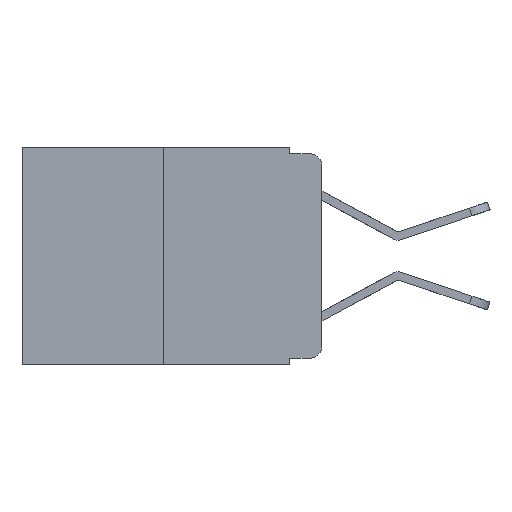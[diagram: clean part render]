
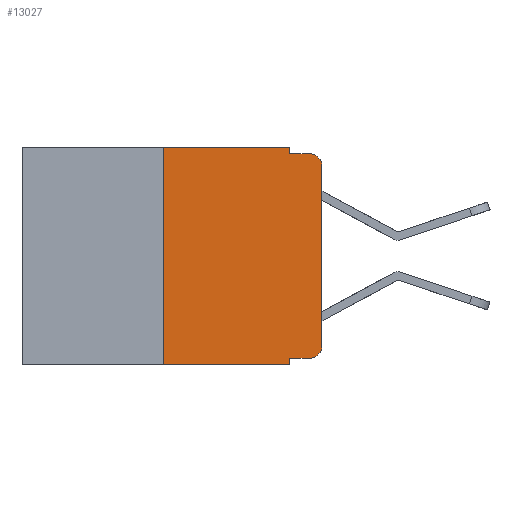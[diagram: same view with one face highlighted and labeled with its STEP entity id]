
A CAD part, left-side view. The second image highlights one B-rep face of the part: STEP entity #13027.
In plain terms, the highlighted planar face has unit normal (-1, 0, 0).
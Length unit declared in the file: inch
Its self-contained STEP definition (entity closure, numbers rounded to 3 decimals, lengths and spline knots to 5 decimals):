
#155 = DIRECTION ( 'NONE',  ( 0., 0., -1. ) ) ;
#633 = EDGE_CURVE ( 'NONE', #12892, #7925, #18901, .T. ) ;
#988 = CARTESIAN_POINT ( 'NONE',  ( 0., 0.473, 0. ) ) ;
#1203 = CARTESIAN_POINT ( 'NONE',  ( 0., 0., -0.313 ) ) ;
#1258 = LINE ( 'NONE', #5531, #10584 ) ;
#1851 = EDGE_CURVE ( 'NONE', #12892, #17118, #18380, .T. ) ;
#2060 = DIRECTION ( 'NONE',  ( 0., -1., 0. ) ) ;
#2754 = CARTESIAN_POINT ( 'NONE',  ( 0., 0.051, 0. ) ) ;
#2759 = ORIENTED_EDGE ( 'NONE', *, *, #19299, .F. ) ;
#2772 = CARTESIAN_POINT ( 'NONE',  ( 0., 0.051, 0. ) ) ;
#2945 = EDGE_CURVE ( 'NONE', #16185, #15703, #11180, .T. ) ;
#3005 = CARTESIAN_POINT ( 'NONE',  ( 0., 0.02, -0.313 ) ) ;
#3011 = VERTEX_POINT ( 'NONE', #1203 ) ;
#3525 = VECTOR ( 'NONE', #8619, 39.37008 ) ;
#3575 = DIRECTION ( 'NONE',  ( -1., 0., 0. ) ) ;
#3885 = CARTESIAN_POINT ( 'NONE',  ( 0., 0.25, 0. ) ) ;
#3967 = ORIENTED_EDGE ( 'NONE', *, *, #5027, .F. ) ;
#3997 = EDGE_CURVE ( 'NONE', #11371, #7748, #6246, .T. ) ;
#4402 = CARTESIAN_POINT ( 'NONE',  ( 0., 0., 0. ) ) ;
#4403 = CARTESIAN_POINT ( 'NONE',  ( 0., 0.051, -0.333 ) ) ;
#4452 = ORIENTED_EDGE ( 'NONE', *, *, #3997, .F. ) ;
#4563 = DIRECTION ( 'NONE',  ( 0., 0., -1. ) ) ;
#4680 = PLANE ( 'NONE',  #9326 ) ;
#5027 = EDGE_CURVE ( 'NONE', #7748, #17074, #13761, .T. ) ;
#5036 = EDGE_LOOP ( 'NONE', ( #16020, #12309, #3967, #4452, #2759, #12347, #14189, #13517, #11882, #10264 ) ) ;
#5135 = LINE ( 'NONE', #4402, #8763 ) ;
#5531 = CARTESIAN_POINT ( 'NONE',  ( 0., 0.473, -0.343 ) ) ;
#6076 = EDGE_CURVE ( 'NONE', #17102, #17074, #17154, .T. ) ;
#6246 = LINE ( 'NONE', #2772, #7215 ) ;
#6347 = AXIS2_PLACEMENT_3D ( 'NONE', #3005, #13666, #4563 ) ;
#6385 = CARTESIAN_POINT ( 'NONE',  ( 0., 0.051, -0.333 ) ) ;
#7058 = CARTESIAN_POINT ( 'NONE',  ( 0., 0.02, -0.01 ) ) ;
#7127 = EDGE_CURVE ( 'NONE', #3011, #17102, #5135, .T. ) ;
#7215 = VECTOR ( 'NONE', #11944, 39.37008 ) ;
#7748 = VERTEX_POINT ( 'NONE', #16337 ) ;
#7925 = VERTEX_POINT ( 'NONE', #18157 ) ;
#8619 = DIRECTION ( 'NONE',  ( 0., 0., 1. ) ) ;
#8664 = CARTESIAN_POINT ( 'NONE',  ( 0., 0., -0.03 ) ) ;
#8763 = VECTOR ( 'NONE', #17907, 39.37008 ) ;
#9131 = CARTESIAN_POINT ( 'NONE',  ( 0., 0.25, -0.343 ) ) ;
#9326 = AXIS2_PLACEMENT_3D ( 'NONE', #13775, #9330, #19650 ) ;
#9330 = DIRECTION ( 'NONE',  ( 1., 0., 0. ) ) ;
#9785 = VECTOR ( 'NONE', #17365, 39.37008 ) ;
#9800 = EDGE_CURVE ( 'NONE', #16185, #17118, #1258, .T. ) ;
#10264 = ORIENTED_EDGE ( 'NONE', *, *, #19422, .T. ) ;
#10584 = VECTOR ( 'NONE', #14583, 39.37008 ) ;
#11081 = VECTOR ( 'NONE', #2060, 39.37008 ) ;
#11180 = LINE ( 'NONE', #3885, #3525 ) ;
#11371 = VERTEX_POINT ( 'NONE', #2754 ) ;
#11882 = ORIENTED_EDGE ( 'NONE', *, *, #633, .T. ) ;
#11944 = DIRECTION ( 'NONE',  ( 0., 0., -1. ) ) ;
#12309 = ORIENTED_EDGE ( 'NONE', *, *, #6076, .T. ) ;
#12347 = ORIENTED_EDGE ( 'NONE', *, *, #2945, .F. ) ;
#12706 = CARTESIAN_POINT ( 'NONE',  ( 0., 0.051, 0. ) ) ;
#12710 = CARTESIAN_POINT ( 'NONE',  ( 0., 0.02, -0.03 ) ) ;
#12892 = VERTEX_POINT ( 'NONE', #4403 ) ;
#13027 = ADVANCED_FACE ( 'NONE', ( #17863 ), #4680, .F. ) ;
#13517 = ORIENTED_EDGE ( 'NONE', *, *, #1851, .F. ) ;
#13666 = DIRECTION ( 'NONE',  ( -1., 0., 0. ) ) ;
#13761 = LINE ( 'NONE', #17633, #9785 ) ;
#13775 = CARTESIAN_POINT ( 'NONE',  ( 0., 0.473, 0. ) ) ;
#14033 = VECTOR ( 'NONE', #155, 39.37008 ) ;
#14056 = CARTESIAN_POINT ( 'NONE',  ( 0., 0.25, 0. ) ) ;
#14181 = DIRECTION ( 'NONE',  ( 0., 0., -1. ) ) ;
#14189 = ORIENTED_EDGE ( 'NONE', *, *, #9800, .T. ) ;
#14583 = DIRECTION ( 'NONE',  ( 0., -1., 0. ) ) ;
#14619 = VECTOR ( 'NONE', #17746, 39.37008 ) ;
#14644 = AXIS2_PLACEMENT_3D ( 'NONE', #12710, #3575, #14181 ) ;
#15703 = VERTEX_POINT ( 'NONE', #14056 ) ;
#16020 = ORIENTED_EDGE ( 'NONE', *, *, #7127, .T. ) ;
#16185 = VERTEX_POINT ( 'NONE', #9131 ) ;
#16337 = CARTESIAN_POINT ( 'NONE',  ( 0., 0.051, -0.01 ) ) ;
#17074 = VERTEX_POINT ( 'NONE', #7058 ) ;
#17102 = VERTEX_POINT ( 'NONE', #8664 ) ;
#17118 = VERTEX_POINT ( 'NONE', #18995 ) ;
#17154 = CIRCLE ( 'NONE', #14644, 0.02 ) ;
#17365 = DIRECTION ( 'NONE',  ( 0., -1., 0. ) ) ;
#17573 = CIRCLE ( 'NONE', #6347, 0.02 ) ;
#17633 = CARTESIAN_POINT ( 'NONE',  ( 0., 0.051, -0.01 ) ) ;
#17746 = DIRECTION ( 'NONE',  ( 0., -1., 0. ) ) ;
#17863 = FACE_OUTER_BOUND ( 'NONE', #5036, .T. ) ;
#17907 = DIRECTION ( 'NONE',  ( 0., 0., 1. ) ) ;
#18157 = CARTESIAN_POINT ( 'NONE',  ( 0., 0.02, -0.333 ) ) ;
#18380 = LINE ( 'NONE', #12706, #14033 ) ;
#18501 = LINE ( 'NONE', #988, #14619 ) ;
#18901 = LINE ( 'NONE', #6385, #11081 ) ;
#18995 = CARTESIAN_POINT ( 'NONE',  ( 0., 0.051, -0.343 ) ) ;
#19299 = EDGE_CURVE ( 'NONE', #15703, #11371, #18501, .T. ) ;
#19422 = EDGE_CURVE ( 'NONE', #7925, #3011, #17573, .T. ) ;
#19650 = DIRECTION ( 'NONE',  ( 0., 0., -1. ) ) ;
